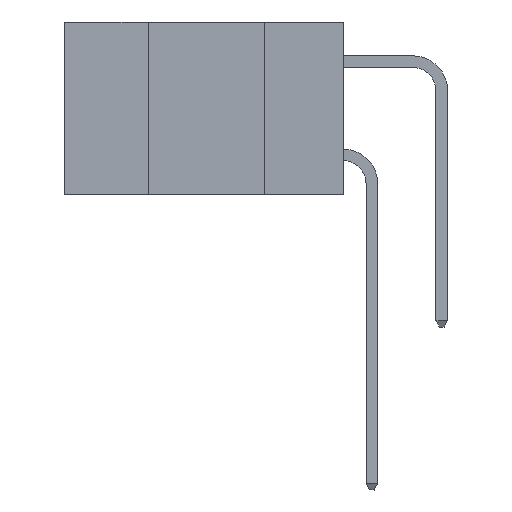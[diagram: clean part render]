
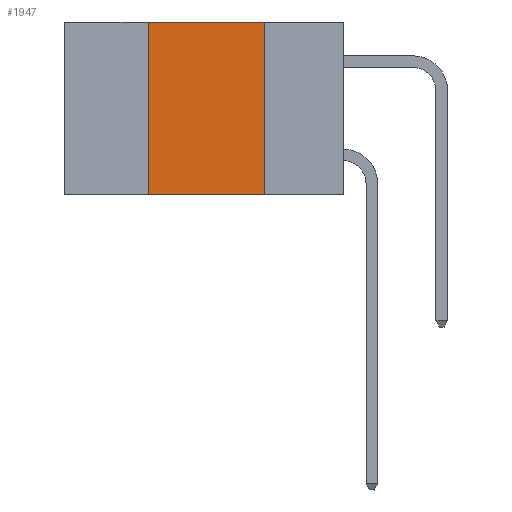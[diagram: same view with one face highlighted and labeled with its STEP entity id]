
A CAD part, left-side view. The second image highlights one B-rep face of the part: STEP entity #1947.
In plain terms, the highlighted planar face has unit normal (-1, 0, 0).
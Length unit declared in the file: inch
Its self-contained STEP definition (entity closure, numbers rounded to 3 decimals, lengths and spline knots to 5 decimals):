
#384 = LINE ( 'NONE', #4737, #10089 ) ;
#463 = EDGE_LOOP ( 'NONE', ( #11949, #13369, #8620, #5999 ) ) ;
#1947 = ADVANCED_FACE ( 'NONE', ( #4949 ), #12202, .F. ) ;
#2115 = EDGE_CURVE ( 'NONE', #5510, #3443, #15862, .T. ) ;
#2210 = CARTESIAN_POINT ( 'NONE',  ( 0., 0.6, 0. ) ) ;
#2264 = CARTESIAN_POINT ( 'NONE',  ( 0., 0.42, -0.37 ) ) ;
#2301 = EDGE_CURVE ( 'NONE', #3443, #14143, #384, .T. ) ;
#3443 = VERTEX_POINT ( 'NONE', #16363 ) ;
#4090 = CARTESIAN_POINT ( 'NONE',  ( 0., 0.6, 0. ) ) ;
#4737 = CARTESIAN_POINT ( 'NONE',  ( 0., 0.17, -0.37 ) ) ;
#4788 = VECTOR ( 'NONE', #16775, 39.37008 ) ;
#4949 = FACE_OUTER_BOUND ( 'NONE', #463, .T. ) ;
#5510 = VERTEX_POINT ( 'NONE', #7203 ) ;
#5999 = ORIENTED_EDGE ( 'NONE', *, *, #16518, .T. ) ;
#7180 = LINE ( 'NONE', #13050, #14389 ) ;
#7203 = CARTESIAN_POINT ( 'NONE',  ( 0., 0.42, 0. ) ) ;
#7439 = EDGE_CURVE ( 'NONE', #10355, #5510, #12068, .T. ) ;
#7484 = DIRECTION ( 'NONE',  ( 0., 0., -1. ) ) ;
#7779 = DIRECTION ( 'NONE',  ( 0., 0., -1. ) ) ;
#8620 = ORIENTED_EDGE ( 'NONE', *, *, #7439, .F. ) ;
#8633 = DIRECTION ( 'NONE',  ( 0., -1., 0. ) ) ;
#9429 = AXIS2_PLACEMENT_3D ( 'NONE', #2210, #13862, #7779 ) ;
#10089 = VECTOR ( 'NONE', #7484, 39.37008 ) ;
#10355 = VERTEX_POINT ( 'NONE', #16869 ) ;
#11568 = VECTOR ( 'NONE', #8633, 39.37008 ) ;
#11949 = ORIENTED_EDGE ( 'NONE', *, *, #2301, .F. ) ;
#12068 = LINE ( 'NONE', #2264, #4788 ) ;
#12202 = PLANE ( 'NONE',  #9429 ) ;
#13050 = CARTESIAN_POINT ( 'NONE',  ( 0., 0.6, -0.37 ) ) ;
#13369 = ORIENTED_EDGE ( 'NONE', *, *, #2115, .F. ) ;
#13862 = DIRECTION ( 'NONE',  ( 1., 0., 0. ) ) ;
#14143 = VERTEX_POINT ( 'NONE', #18540 ) ;
#14389 = VECTOR ( 'NONE', #17163, 39.37008 ) ;
#15862 = LINE ( 'NONE', #4090, #11568 ) ;
#16363 = CARTESIAN_POINT ( 'NONE',  ( 0., 0.17, 0. ) ) ;
#16518 = EDGE_CURVE ( 'NONE', #10355, #14143, #7180, .T. ) ;
#16775 = DIRECTION ( 'NONE',  ( 0., 0., 1. ) ) ;
#16869 = CARTESIAN_POINT ( 'NONE',  ( 0., 0.42, -0.37 ) ) ;
#17163 = DIRECTION ( 'NONE',  ( 0., -1., 0. ) ) ;
#18540 = CARTESIAN_POINT ( 'NONE',  ( 0., 0.17, -0.37 ) ) ;
